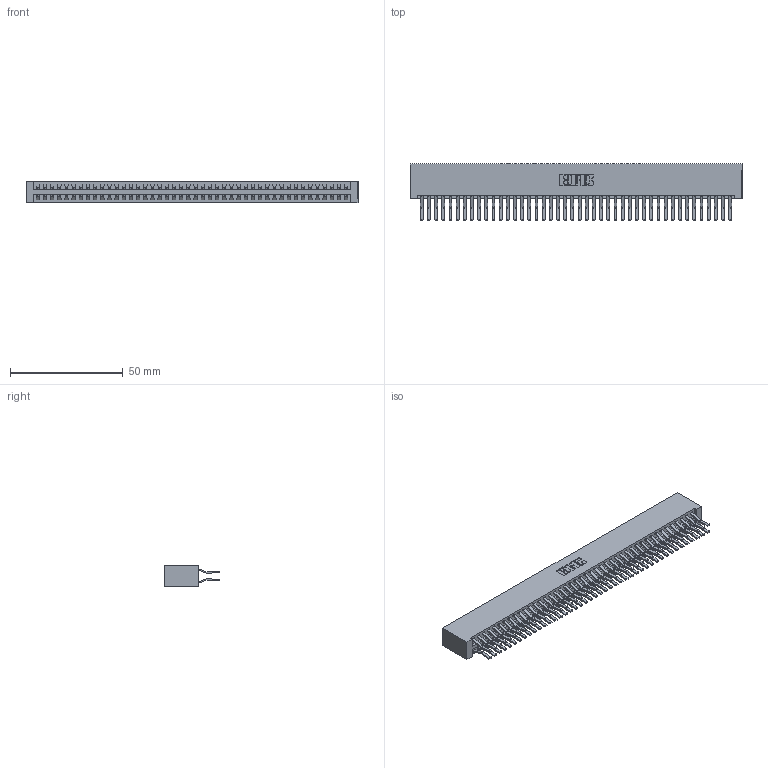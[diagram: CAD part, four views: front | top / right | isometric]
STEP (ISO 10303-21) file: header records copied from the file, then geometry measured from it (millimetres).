
FILE_DESCRIPTION (( 'STEP AP203' ), '1' );
FILE_NAME ('346-088-560-201.STEP', '2022-05-26T02:30:11', ( '' ), ( '' ), 'SwSTEP 2.0', 'SolidWorks 2020', '' );
FILE_SCHEMA (( 'CONFIG_CONTROL_DESIGN' ));
Length unit declared in the file: inch
Products named in the file (3): 346-088-560-201; 345-292-001_560 Tail; 346 Part_No Mounting Lugs
Assembly tree (89 placements, depth 2):
  346-088-560-201
    346 Part_No Mounting Lugs
    345-292-001_560 Tail  x88
Bounding box: 146.94 x 24.78 x 9.4 mm (x, y, z)
Volume: 15494 mm3; surface area: 23031.1 mm2
Topology: 89 solids, 89 shells, 4866 faces, 14473 edges, 9530 vertices
Faces by surface type: plane 3152, cylinder 1714
Entity records: 28257 total; most frequent: CARTESIAN_POINT 4652, ORIENTED_EDGE 4586, DIRECTION 4149, EDGE_CURVE 2293, VECTOR 1989, LINE 1989, VERTEX_POINT 1526, AXIS2_PLACEMENT_3D 1080
